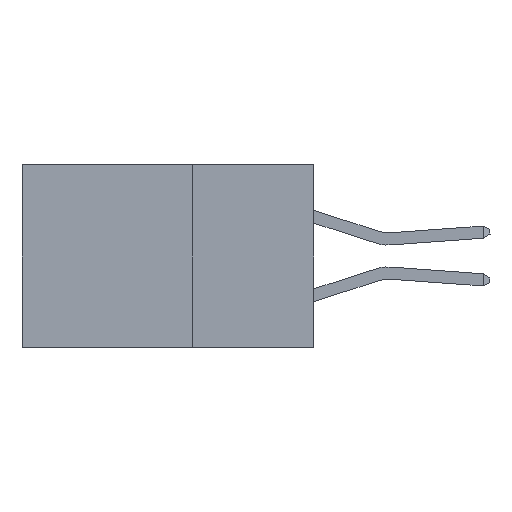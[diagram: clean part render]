
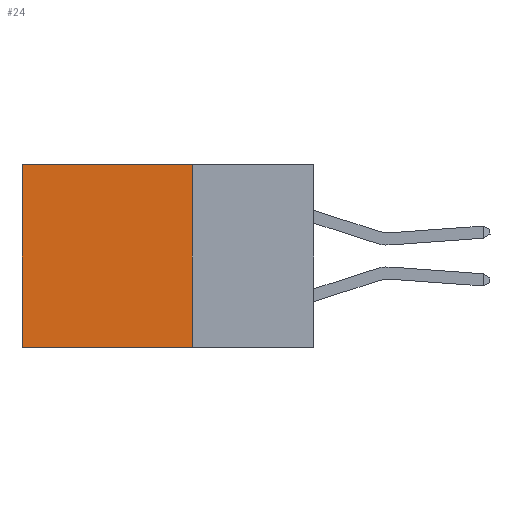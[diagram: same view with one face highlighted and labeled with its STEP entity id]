
A CAD part, left-side view. The second image highlights one B-rep face of the part: STEP entity #24.
In plain terms, the highlighted planar face has unit normal (-1, 0, 0).
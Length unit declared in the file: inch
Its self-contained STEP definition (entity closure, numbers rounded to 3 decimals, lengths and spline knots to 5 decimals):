
#24 = ADVANCED_FACE ( 'NONE', ( #4871 ), #5033, .F. ) ;
#82 = DIRECTION ( 'NONE',  ( 1., 0., 0. ) ) ;
#187 = EDGE_CURVE ( 'NONE', #3612, #938, #6013, .T. ) ;
#539 = LINE ( 'NONE', #7143, #865 ) ;
#689 = DIRECTION ( 'NONE',  ( 0., 0., -1. ) ) ;
#736 = LINE ( 'NONE', #7844, #7388 ) ;
#865 = VECTOR ( 'NONE', #3254, 39.37008 ) ;
#938 = VERTEX_POINT ( 'NONE', #2056 ) ;
#1200 = CARTESIAN_POINT ( 'NONE',  ( 0.2875, 0.25, -0.375 ) ) ;
#1305 = CARTESIAN_POINT ( 'NONE',  ( 0.2875, 0.25, -0.375 ) ) ;
#1550 = CARTESIAN_POINT ( 'NONE',  ( 0.2875, 0.25, -0.375 ) ) ;
#1967 = CARTESIAN_POINT ( 'NONE',  ( 0.2875, 0.25, 0. ) ) ;
#1993 = EDGE_CURVE ( 'NONE', #6950, #938, #539, .T. ) ;
#2056 = CARTESIAN_POINT ( 'NONE',  ( 0.2875, 0.6, -0.375 ) ) ;
#2149 = DIRECTION ( 'NONE',  ( 0., 0., -1. ) ) ;
#2689 = AXIS2_PLACEMENT_3D ( 'NONE', #1200, #82, #2149 ) ;
#2869 = EDGE_LOOP ( 'NONE', ( #3849, #6848, #4772, #4067 ) ) ;
#3254 = DIRECTION ( 'NONE',  ( 0., 1., 0. ) ) ;
#3323 = LINE ( 'NONE', #1305, #7168 ) ;
#3526 = CARTESIAN_POINT ( 'NONE',  ( 0.2875, 0.6, 0. ) ) ;
#3612 = VERTEX_POINT ( 'NONE', #3526 ) ;
#3849 = ORIENTED_EDGE ( 'NONE', *, *, #187, .T. ) ;
#4067 = ORIENTED_EDGE ( 'NONE', *, *, #7923, .T. ) ;
#4169 = EDGE_CURVE ( 'NONE', #8377, #6950, #3323, .T. ) ;
#4522 = DIRECTION ( 'NONE',  ( 0., 1., 0. ) ) ;
#4659 = VECTOR ( 'NONE', #5008, 39.37008 ) ;
#4772 = ORIENTED_EDGE ( 'NONE', *, *, #4169, .F. ) ;
#4871 = FACE_OUTER_BOUND ( 'NONE', #2869, .T. ) ;
#5008 = DIRECTION ( 'NONE',  ( 0., 0., -1. ) ) ;
#5033 = PLANE ( 'NONE',  #2689 ) ;
#6013 = LINE ( 'NONE', #7987, #4659 ) ;
#6848 = ORIENTED_EDGE ( 'NONE', *, *, #1993, .F. ) ;
#6950 = VERTEX_POINT ( 'NONE', #1550 ) ;
#7143 = CARTESIAN_POINT ( 'NONE',  ( 0.2875, 0.25, -0.375 ) ) ;
#7168 = VECTOR ( 'NONE', #689, 39.37008 ) ;
#7388 = VECTOR ( 'NONE', #4522, 39.37008 ) ;
#7844 = CARTESIAN_POINT ( 'NONE',  ( 0.2875, 0.25, 0. ) ) ;
#7923 = EDGE_CURVE ( 'NONE', #8377, #3612, #736, .T. ) ;
#7987 = CARTESIAN_POINT ( 'NONE',  ( 0.2875, 0.6, -0.375 ) ) ;
#8377 = VERTEX_POINT ( 'NONE', #1967 ) ;
